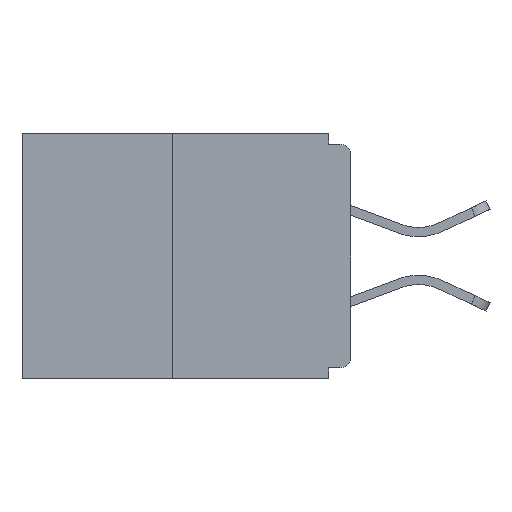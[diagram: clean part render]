
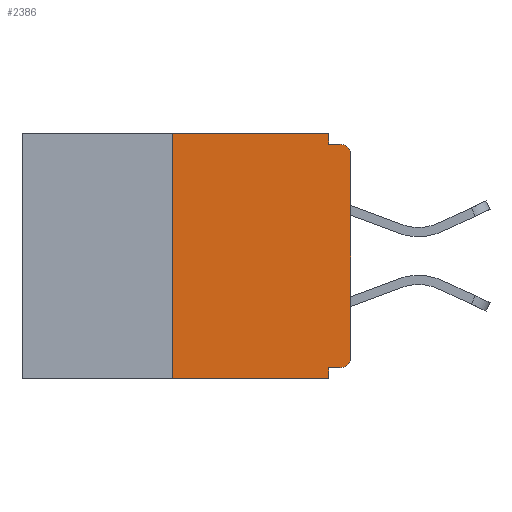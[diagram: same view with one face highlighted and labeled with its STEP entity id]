
A CAD part, left-side view. The second image highlights one B-rep face of the part: STEP entity #2386.
In plain terms, the highlighted planar face has unit normal (-1, 0, 0).
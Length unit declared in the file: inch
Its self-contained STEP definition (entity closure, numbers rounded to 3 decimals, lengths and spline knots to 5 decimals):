
#20 = VERTEX_POINT ( 'NONE', #11876 ) ;
#37 = CARTESIAN_POINT ( 'NONE',  ( 0., 0., -0.313 ) ) ;
#183 = VECTOR ( 'NONE', #12140, 39.37008 ) ;
#238 = VECTOR ( 'NONE', #12933, 39.37008 ) ;
#1436 = CARTESIAN_POINT ( 'NONE',  ( 0., 0.031, -0.328 ) ) ;
#1566 = CARTESIAN_POINT ( 'NONE',  ( 0., 0.015, -0.03 ) ) ;
#1849 = CIRCLE ( 'NONE', #6549, 0.015 ) ;
#2264 = DIRECTION ( 'NONE',  ( 0., 0., -1. ) ) ;
#2386 = ADVANCED_FACE ( 'NONE', ( #2440 ), #12405, .F. ) ;
#2440 = FACE_OUTER_BOUND ( 'NONE', #14541, .T. ) ;
#2523 = CARTESIAN_POINT ( 'NONE',  ( 0., 0., -0.015 ) ) ;
#2827 = VERTEX_POINT ( 'NONE', #6479 ) ;
#3085 = CIRCLE ( 'NONE', #9864, 0.015 ) ;
#3261 = EDGE_CURVE ( 'NONE', #4442, #15468, #3864, .T. ) ;
#3468 = CARTESIAN_POINT ( 'NONE',  ( 0., 0.015, -0.313 ) ) ;
#3864 = LINE ( 'NONE', #14846, #5506 ) ;
#3904 = LINE ( 'NONE', #2523, #17002 ) ;
#3948 = CARTESIAN_POINT ( 'NONE',  ( 0., 0., -0.328 ) ) ;
#4426 = EDGE_CURVE ( 'NONE', #5480, #12667, #6637, .T. ) ;
#4442 = VERTEX_POINT ( 'NONE', #16606 ) ;
#4604 = EDGE_CURVE ( 'NONE', #8353, #12667, #7286, .T. ) ;
#4988 = ORIENTED_EDGE ( 'NONE', *, *, #3261, .F. ) ;
#4999 = ORIENTED_EDGE ( 'NONE', *, *, #8927, .T. ) ;
#5333 = LINE ( 'NONE', #3948, #10040 ) ;
#5360 = ORIENTED_EDGE ( 'NONE', *, *, #4604, .T. ) ;
#5480 = VERTEX_POINT ( 'NONE', #1436 ) ;
#5506 = VECTOR ( 'NONE', #6354, 39.37008 ) ;
#5912 = EDGE_CURVE ( 'NONE', #8775, #4442, #14593, .T. ) ;
#6354 = DIRECTION ( 'NONE',  ( 0., 0., -1. ) ) ;
#6479 = CARTESIAN_POINT ( 'NONE',  ( 0., 0.015, -0.015 ) ) ;
#6549 = AXIS2_PLACEMENT_3D ( 'NONE', #3468, #17858, #2264 ) ;
#6637 = LINE ( 'NONE', #12373, #11146 ) ;
#6663 = AXIS2_PLACEMENT_3D ( 'NONE', #14896, #16377, #7895 ) ;
#6873 = EDGE_CURVE ( 'NONE', #8793, #13610, #1849, .T. ) ;
#7020 = ORIENTED_EDGE ( 'NONE', *, *, #5912, .F. ) ;
#7286 = LINE ( 'NONE', #8938, #238 ) ;
#7812 = EDGE_CURVE ( 'NONE', #8793, #5480, #5333, .T. ) ;
#7871 = EDGE_CURVE ( 'NONE', #8353, #8775, #16690, .T. ) ;
#7895 = DIRECTION ( 'NONE',  ( 0., 0., -1. ) ) ;
#8353 = VERTEX_POINT ( 'NONE', #14338 ) ;
#8775 = VERTEX_POINT ( 'NONE', #14695 ) ;
#8793 = VERTEX_POINT ( 'NONE', #12376 ) ;
#8868 = VECTOR ( 'NONE', #10885, 39.37008 ) ;
#8927 = EDGE_CURVE ( 'NONE', #20, #2827, #3085, .T. ) ;
#8938 = CARTESIAN_POINT ( 'NONE',  ( 0., 0.46, -0.343 ) ) ;
#9056 = CARTESIAN_POINT ( 'NONE',  ( 0., 0.46, 0. ) ) ;
#9530 = DIRECTION ( 'NONE',  ( 0., -1., 0. ) ) ;
#9864 = AXIS2_PLACEMENT_3D ( 'NONE', #1566, #15865, #14211 ) ;
#10040 = VECTOR ( 'NONE', #16602, 39.37008 ) ;
#10109 = ORIENTED_EDGE ( 'NONE', *, *, #4426, .F. ) ;
#10617 = ORIENTED_EDGE ( 'NONE', *, *, #7871, .F. ) ;
#10654 = LINE ( 'NONE', #11867, #183 ) ;
#10722 = EDGE_CURVE ( 'NONE', #13610, #20, #10654, .T. ) ;
#10885 = DIRECTION ( 'NONE',  ( 0., 0., 1. ) ) ;
#10924 = EDGE_CURVE ( 'NONE', #15468, #2827, #3904, .T. ) ;
#10938 = VECTOR ( 'NONE', #12019, 39.37008 ) ;
#11146 = VECTOR ( 'NONE', #18079, 39.37008 ) ;
#11867 = CARTESIAN_POINT ( 'NONE',  ( 0., 0., 0. ) ) ;
#11876 = CARTESIAN_POINT ( 'NONE',  ( 0., 0., -0.03 ) ) ;
#12019 = DIRECTION ( 'NONE',  ( 0., -1., 0. ) ) ;
#12140 = DIRECTION ( 'NONE',  ( 0., 0., 1. ) ) ;
#12201 = CARTESIAN_POINT ( 'NONE',  ( 0., 0.031, -0.015 ) ) ;
#12373 = CARTESIAN_POINT ( 'NONE',  ( 0., 0.031, -0.343 ) ) ;
#12376 = CARTESIAN_POINT ( 'NONE',  ( 0., 0.015, -0.328 ) ) ;
#12405 = PLANE ( 'NONE',  #6663 ) ;
#12667 = VERTEX_POINT ( 'NONE', #15225 ) ;
#12933 = DIRECTION ( 'NONE',  ( 0., -1., 0. ) ) ;
#13314 = ORIENTED_EDGE ( 'NONE', *, *, #6873, .T. ) ;
#13610 = VERTEX_POINT ( 'NONE', #37 ) ;
#14063 = ORIENTED_EDGE ( 'NONE', *, *, #10722, .T. ) ;
#14211 = DIRECTION ( 'NONE',  ( 0., 0., -1. ) ) ;
#14338 = CARTESIAN_POINT ( 'NONE',  ( 0., 0.25, -0.343 ) ) ;
#14541 = EDGE_LOOP ( 'NONE', ( #7020, #10617, #5360, #10109, #15377, #13314, #14063, #4999, #16130, #4988 ) ) ;
#14593 = LINE ( 'NONE', #9056, #10938 ) ;
#14695 = CARTESIAN_POINT ( 'NONE',  ( 0., 0.25, 0. ) ) ;
#14846 = CARTESIAN_POINT ( 'NONE',  ( 0., 0.031, 0. ) ) ;
#14896 = CARTESIAN_POINT ( 'NONE',  ( 0., 0.46, 0. ) ) ;
#15225 = CARTESIAN_POINT ( 'NONE',  ( 0., 0.031, -0.343 ) ) ;
#15377 = ORIENTED_EDGE ( 'NONE', *, *, #7812, .F. ) ;
#15468 = VERTEX_POINT ( 'NONE', #12201 ) ;
#15865 = DIRECTION ( 'NONE',  ( -1., 0., 0. ) ) ;
#16130 = ORIENTED_EDGE ( 'NONE', *, *, #10924, .F. ) ;
#16377 = DIRECTION ( 'NONE',  ( 1., 0., 0. ) ) ;
#16602 = DIRECTION ( 'NONE',  ( 0., 1., 0. ) ) ;
#16606 = CARTESIAN_POINT ( 'NONE',  ( 0., 0.031, 0. ) ) ;
#16690 = LINE ( 'NONE', #18165, #8868 ) ;
#17002 = VECTOR ( 'NONE', #9530, 39.37008 ) ;
#17858 = DIRECTION ( 'NONE',  ( -1., 0., 0. ) ) ;
#18079 = DIRECTION ( 'NONE',  ( 0., 0., -1. ) ) ;
#18165 = CARTESIAN_POINT ( 'NONE',  ( 0., 0.25, 0. ) ) ;
